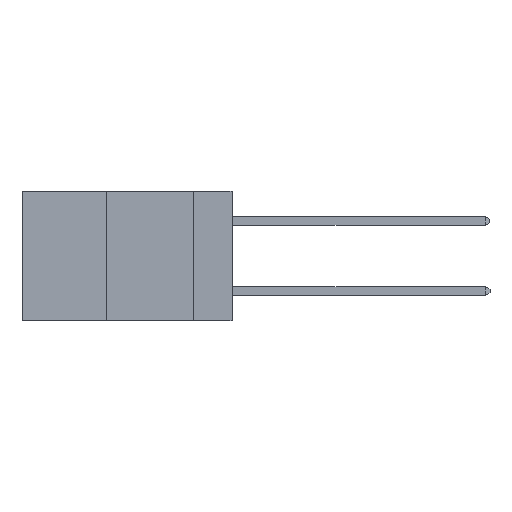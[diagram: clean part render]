
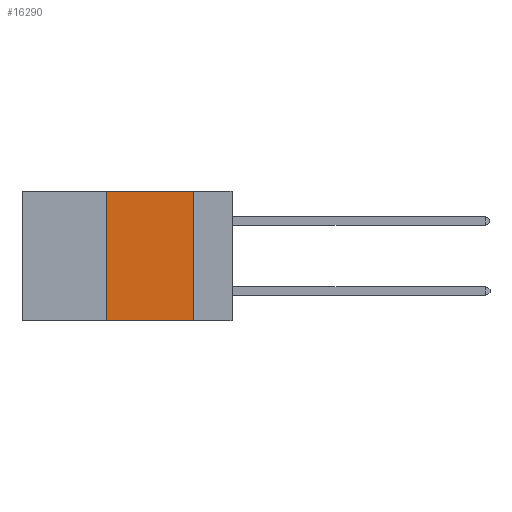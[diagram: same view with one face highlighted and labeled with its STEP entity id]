
A CAD part, left-side view. The second image highlights one B-rep face of the part: STEP entity #16290.
In plain terms, the highlighted planar face has unit normal (-1, 0, 0).
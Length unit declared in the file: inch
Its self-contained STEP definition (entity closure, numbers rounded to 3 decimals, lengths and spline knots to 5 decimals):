
#641 = VERTEX_POINT ( 'NONE', #11429 ) ;
#1129 = CARTESIAN_POINT ( 'NONE',  ( 0., 0.6, -0.37 ) ) ;
#1685 = VECTOR ( 'NONE', #3130, 39.37008 ) ;
#1744 = EDGE_CURVE ( 'NONE', #9708, #641, #19560, .T. ) ;
#2349 = DIRECTION ( 'NONE',  ( 0., 0., 1. ) ) ;
#3130 = DIRECTION ( 'NONE',  ( 0., -1., 0. ) ) ;
#3566 = CARTESIAN_POINT ( 'NONE',  ( 0., 0.6, 0. ) ) ;
#5068 = CARTESIAN_POINT ( 'NONE',  ( 0., 0.36, -0.37 ) ) ;
#5210 = EDGE_CURVE ( 'NONE', #13862, #9708, #11510, .T. ) ;
#6659 = ORIENTED_EDGE ( 'NONE', *, *, #10669, .T. ) ;
#7301 = DIRECTION ( 'NONE',  ( 1., 0., 0. ) ) ;
#8189 = FACE_OUTER_BOUND ( 'NONE', #23319, .T. ) ;
#8868 = CARTESIAN_POINT ( 'NONE',  ( 0., 0.36, 0. ) ) ;
#9708 = VERTEX_POINT ( 'NONE', #8868 ) ;
#10669 = EDGE_CURVE ( 'NONE', #13862, #14209, #11644, .T. ) ;
#10948 = VECTOR ( 'NONE', #2349, 39.37008 ) ;
#11429 = CARTESIAN_POINT ( 'NONE',  ( 0., 0.11, 0. ) ) ;
#11510 = LINE ( 'NONE', #11653, #10948 ) ;
#11530 = CARTESIAN_POINT ( 'NONE',  ( 0., 0.11, -0.37 ) ) ;
#11644 = LINE ( 'NONE', #1129, #1685 ) ;
#11653 = CARTESIAN_POINT ( 'NONE',  ( 0., 0.36, 0. ) ) ;
#12614 = ORIENTED_EDGE ( 'NONE', *, *, #1744, .F. ) ;
#12693 = AXIS2_PLACEMENT_3D ( 'NONE', #18012, #7301, #19791 ) ;
#12895 = ORIENTED_EDGE ( 'NONE', *, *, #5210, .F. ) ;
#13862 = VERTEX_POINT ( 'NONE', #5068 ) ;
#14209 = VERTEX_POINT ( 'NONE', #11530 ) ;
#14451 = PLANE ( 'NONE',  #12693 ) ;
#14783 = ORIENTED_EDGE ( 'NONE', *, *, #20884, .F. ) ;
#16290 = ADVANCED_FACE ( 'NONE', ( #8189 ), #14451, .F. ) ;
#17300 = CARTESIAN_POINT ( 'NONE',  ( 0., 0.11, 0. ) ) ;
#17728 = LINE ( 'NONE', #17300, #21832 ) ;
#18012 = CARTESIAN_POINT ( 'NONE',  ( 0., 0.6, 0. ) ) ;
#19560 = LINE ( 'NONE', #3566, #23076 ) ;
#19791 = DIRECTION ( 'NONE',  ( 0., 0., -1. ) ) ;
#20884 = EDGE_CURVE ( 'NONE', #641, #14209, #17728, .T. ) ;
#21832 = VECTOR ( 'NONE', #22572, 39.37008 ) ;
#22572 = DIRECTION ( 'NONE',  ( 0., 0., -1. ) ) ;
#23076 = VECTOR ( 'NONE', #23325, 39.37008 ) ;
#23319 = EDGE_LOOP ( 'NONE', ( #14783, #12614, #12895, #6659 ) ) ;
#23325 = DIRECTION ( 'NONE',  ( 0., -1., 0. ) ) ;
